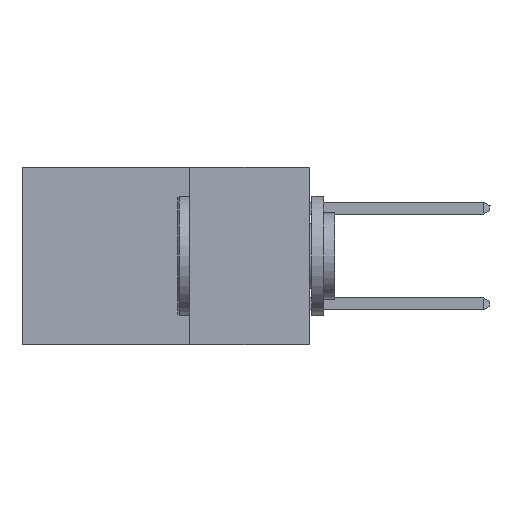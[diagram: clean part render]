
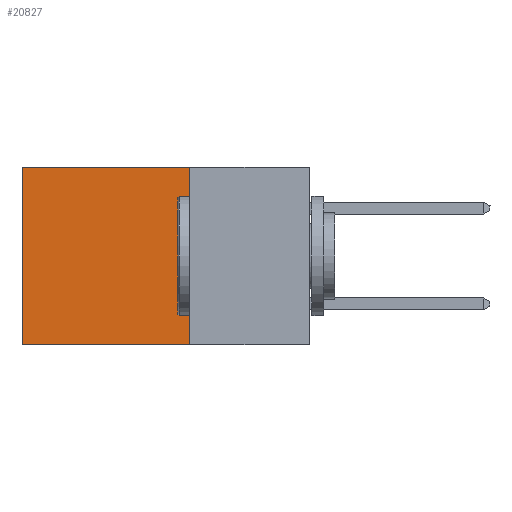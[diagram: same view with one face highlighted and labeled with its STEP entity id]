
A CAD part, left-side view. The second image highlights one B-rep face of the part: STEP entity #20827.
In plain terms, the highlighted planar face has unit normal (-1, 0, 0).
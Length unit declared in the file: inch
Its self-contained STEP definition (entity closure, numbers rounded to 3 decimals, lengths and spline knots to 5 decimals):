
#851 = DIRECTION ( 'NONE',  ( 1., 0., 0. ) ) ;
#1209 = CARTESIAN_POINT ( 'NONE',  ( 0.2875, 0.25, 0. ) ) ;
#2625 = LINE ( 'NONE', #22874, #28080 ) ;
#3542 = ORIENTED_EDGE ( 'NONE', *, *, #39133, .F. ) ;
#6665 = ORIENTED_EDGE ( 'NONE', *, *, #41455, .T. ) ;
#7541 = EDGE_CURVE ( 'NONE', #26596, #28137, #39204, .T. ) ;
#7589 = ORIENTED_EDGE ( 'NONE', *, *, #21299, .T. ) ;
#7750 = EDGE_LOOP ( 'NONE', ( #7589, #40219, #3542, #6665 ) ) ;
#8709 = CARTESIAN_POINT ( 'NONE',  ( 0.2875, 0.25, 0. ) ) ;
#14542 = AXIS2_PLACEMENT_3D ( 'NONE', #20720, #851, #24074 ) ;
#14687 = DIRECTION ( 'NONE',  ( 0., 1., 0. ) ) ;
#15068 = CARTESIAN_POINT ( 'NONE',  ( 0.2875, 0.25, -0.37 ) ) ;
#16648 = VECTOR ( 'NONE', #14687, 39.37008 ) ;
#16840 = VECTOR ( 'NONE', #37621, 39.37008 ) ;
#17700 = VERTEX_POINT ( 'NONE', #38575 ) ;
#20096 = CARTESIAN_POINT ( 'NONE',  ( 0.2875, 0.6, -0.37 ) ) ;
#20720 = CARTESIAN_POINT ( 'NONE',  ( 0.2875, 0.25, 0. ) ) ;
#20827 = ADVANCED_FACE ( 'NONE', ( #35815 ), #27270, .F. ) ;
#21135 = CARTESIAN_POINT ( 'NONE',  ( 0.2875, 0.25, 0. ) ) ;
#21299 = EDGE_CURVE ( 'NONE', #17700, #28137, #2625, .T. ) ;
#22874 = CARTESIAN_POINT ( 'NONE',  ( 0.2875, 0.6, 0. ) ) ;
#24074 = DIRECTION ( 'NONE',  ( 0., 0., -1. ) ) ;
#25436 = LINE ( 'NONE', #21135, #16648 ) ;
#26596 = VERTEX_POINT ( 'NONE', #38605 ) ;
#27270 = PLANE ( 'NONE',  #14542 ) ;
#27859 = VERTEX_POINT ( 'NONE', #8709 ) ;
#28080 = VECTOR ( 'NONE', #36114, 39.37008 ) ;
#28137 = VERTEX_POINT ( 'NONE', #20096 ) ;
#30550 = VECTOR ( 'NONE', #31511, 39.37008 ) ;
#31511 = DIRECTION ( 'NONE',  ( 0., 1., 0. ) ) ;
#35379 = LINE ( 'NONE', #1209, #16840 ) ;
#35815 = FACE_OUTER_BOUND ( 'NONE', #7750, .T. ) ;
#36114 = DIRECTION ( 'NONE',  ( 0., 0., -1. ) ) ;
#37621 = DIRECTION ( 'NONE',  ( 0., 0., -1. ) ) ;
#38575 = CARTESIAN_POINT ( 'NONE',  ( 0.2875, 0.6, 0. ) ) ;
#38605 = CARTESIAN_POINT ( 'NONE',  ( 0.2875, 0.25, -0.37 ) ) ;
#39133 = EDGE_CURVE ( 'NONE', #27859, #26596, #35379, .T. ) ;
#39204 = LINE ( 'NONE', #15068, #30550 ) ;
#40219 = ORIENTED_EDGE ( 'NONE', *, *, #7541, .F. ) ;
#41455 = EDGE_CURVE ( 'NONE', #27859, #17700, #25436, .T. ) ;
